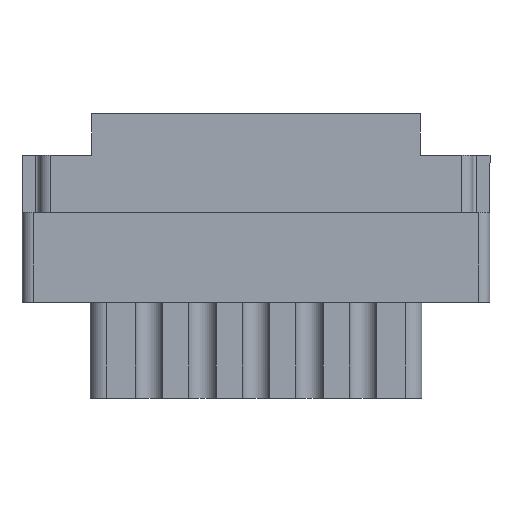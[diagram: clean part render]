
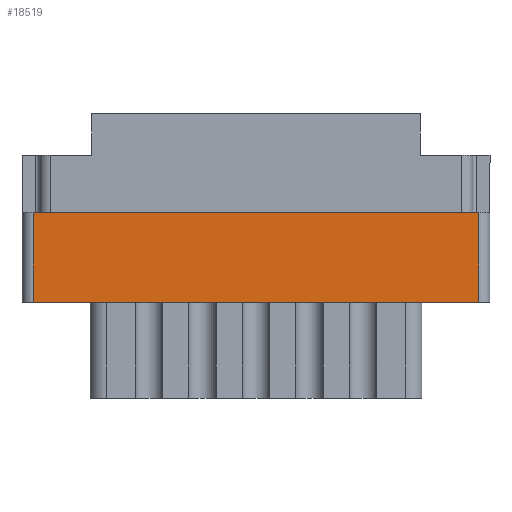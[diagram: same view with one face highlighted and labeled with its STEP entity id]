
A CAD part, front view. The second image highlights one B-rep face of the part: STEP entity #18519.
In plain terms, the highlighted planar face has unit normal (0, -1, 0).
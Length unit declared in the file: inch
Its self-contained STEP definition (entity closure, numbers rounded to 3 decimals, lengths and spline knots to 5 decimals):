
#177 = DIRECTION ( 'NONE',  ( 0., 0., 1. ) ) ;
#250 = VERTEX_POINT ( 'NONE', #3428 ) ;
#278 = LINE ( 'NONE', #1931, #19404 ) ;
#1348 = DIRECTION ( 'NONE',  ( 0., 0., -1. ) ) ;
#1393 = VECTOR ( 'NONE', #19134, 39.37008 ) ;
#1454 = DIRECTION ( 'NONE',  ( -1., 0., 0. ) ) ;
#1600 = AXIS2_PLACEMENT_3D ( 'NONE', #12347, #9232, #1348 ) ;
#1709 = LINE ( 'NONE', #8033, #1393 ) ;
#1931 = CARTESIAN_POINT ( 'NONE',  ( -0.624, -0.343, -0.798 ) ) ;
#2317 = EDGE_LOOP ( 'NONE', ( #4264, #5505, #6136, #7849 ) ) ;
#3007 = CARTESIAN_POINT ( 'NONE',  ( 0.624, -0.343, -0.529 ) ) ;
#3428 = CARTESIAN_POINT ( 'NONE',  ( -0.624, -0.343, -0.529 ) ) ;
#4264 = ORIENTED_EDGE ( 'NONE', *, *, #7966, .F. ) ;
#4330 = CARTESIAN_POINT ( 'NONE',  ( 0.624, -0.343, -0.277 ) ) ;
#5505 = ORIENTED_EDGE ( 'NONE', *, *, #18606, .F. ) ;
#5550 = VECTOR ( 'NONE', #1454, 39.37008 ) ;
#6136 = ORIENTED_EDGE ( 'NONE', *, *, #12588, .T. ) ;
#6563 = LINE ( 'NONE', #11430, #18174 ) ;
#6564 = CARTESIAN_POINT ( 'NONE',  ( -0.624, -0.343, -0.277 ) ) ;
#7084 = EDGE_CURVE ( 'NONE', #9878, #13073, #1709, .T. ) ;
#7849 = ORIENTED_EDGE ( 'NONE', *, *, #7084, .F. ) ;
#7893 = PLANE ( 'NONE',  #1600 ) ;
#7966 = EDGE_CURVE ( 'NONE', #250, #9878, #278, .T. ) ;
#8033 = CARTESIAN_POINT ( 'NONE',  ( -0.656, -0.343, -0.277 ) ) ;
#8867 = VERTEX_POINT ( 'NONE', #14246 ) ;
#9232 = DIRECTION ( 'NONE',  ( 0., -1., 0. ) ) ;
#9878 = VERTEX_POINT ( 'NONE', #6564 ) ;
#10892 = LINE ( 'NONE', #3007, #5550 ) ;
#11430 = CARTESIAN_POINT ( 'NONE',  ( 0.624, -0.343, -0.798 ) ) ;
#12347 = CARTESIAN_POINT ( 'NONE',  ( -0.624, -0.343, -0.798 ) ) ;
#12588 = EDGE_CURVE ( 'NONE', #8867, #13073, #6563, .T. ) ;
#13073 = VERTEX_POINT ( 'NONE', #4330 ) ;
#14003 = FACE_OUTER_BOUND ( 'NONE', #2317, .T. ) ;
#14246 = CARTESIAN_POINT ( 'NONE',  ( 0.624, -0.343, -0.529 ) ) ;
#17751 = DIRECTION ( 'NONE',  ( 0., 0., 1. ) ) ;
#18174 = VECTOR ( 'NONE', #17751, 39.37008 ) ;
#18519 = ADVANCED_FACE ( 'NONE', ( #14003 ), #7893, .T. ) ;
#18606 = EDGE_CURVE ( 'NONE', #8867, #250, #10892, .T. ) ;
#19134 = DIRECTION ( 'NONE',  ( 1., 0., 0. ) ) ;
#19404 = VECTOR ( 'NONE', #177, 39.37008 ) ;
